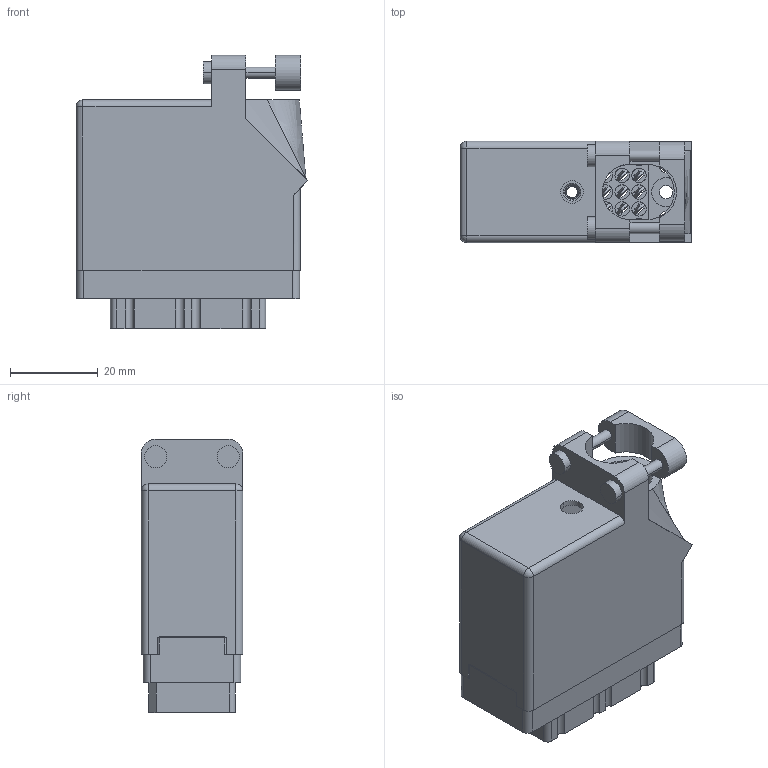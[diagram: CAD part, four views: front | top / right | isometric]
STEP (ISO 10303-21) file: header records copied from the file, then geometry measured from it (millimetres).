
FILE_DESCRIPTION (( 'STEP AP203' ), '1' );
FILE_NAME ('519-036-540-416.STEP', '2020-09-09T21:49:32', ( '' ), ( '' ), 'SwSTEP 2.0', 'SolidWorks 2020', '' );
FILE_SCHEMA (( 'CONFIG_CONTROL_DESIGN' ));
Length unit declared in the file: inch
Products named in the file (5): 519 Receptacle Insulator_036; 519-036-540-416; 516-292-001_540 Contact; 516-230-001_Plastic - 038 Top Entry; 516-252-035-100_516-252-035-100
Assembly tree (39 placements, depth 2):
  519-036-540-416
    519 Receptacle Insulator_036
    516-292-001_540 Contact  x36
    516-252-035-100_516-252-035-100
    516-230-001_Plastic - 038 Top Entry
Bounding box: 52.85 x 23.11 x 62.26 mm (x, y, z)
Volume: 23451.3 mm3; surface area: 35891.2 mm2
Topology: 39 solids, 39 shells, 3563 faces, 10297 edges, 6834 vertices
Faces by surface type: plane 2171, cylinder 1153, bspline 225, cone 12, sphere 2
Entity records: 38674 total; most frequent: CARTESIAN_POINT 8928, ORIENTED_EDGE 6030, DIRECTION 5816, EDGE_CURVE 3015, LINE 2178, VECTOR 2178, VERTEX_POINT 2004, AXIS2_PLACEMENT_3D 1819
